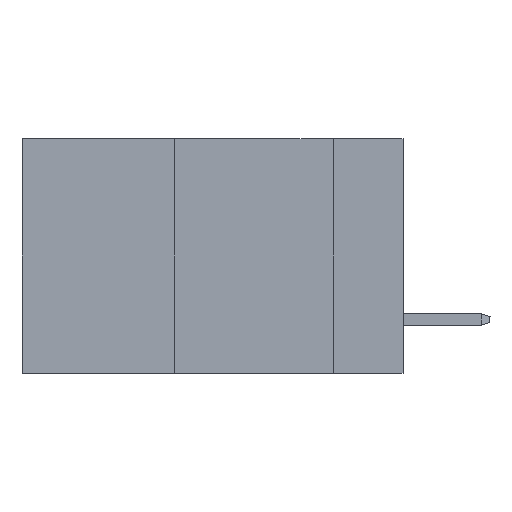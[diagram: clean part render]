
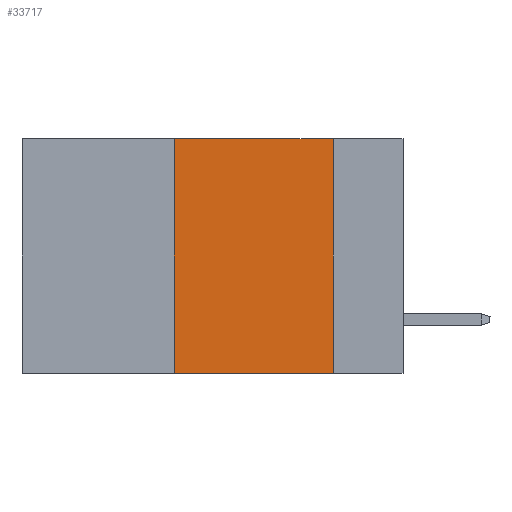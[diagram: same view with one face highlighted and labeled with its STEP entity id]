
A CAD part, left-side view. The second image highlights one B-rep face of the part: STEP entity #33717.
In plain terms, the highlighted planar face has unit normal (-1, 0, 0).
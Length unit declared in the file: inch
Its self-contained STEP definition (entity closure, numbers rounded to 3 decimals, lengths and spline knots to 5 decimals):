
#61 = VECTOR ( 'NONE', #30044, 39.37008 ) ;
#2435 = PLANE ( 'NONE',  #6922 ) ;
#2990 = FACE_OUTER_BOUND ( 'NONE', #19179, .T. ) ;
#3526 = VERTEX_POINT ( 'NONE', #31334 ) ;
#5348 = LINE ( 'NONE', #14117, #12496 ) ;
#5813 = CARTESIAN_POINT ( 'NONE',  ( 0., 0.36, -0.37 ) ) ;
#6833 = VECTOR ( 'NONE', #10161, 39.37008 ) ;
#6896 = CARTESIAN_POINT ( 'NONE',  ( 0., 0.11, 0. ) ) ;
#6922 = AXIS2_PLACEMENT_3D ( 'NONE', #34213, #17043, #23262 ) ;
#7102 = EDGE_CURVE ( 'NONE', #29738, #3526, #18357, .T. ) ;
#7328 = CARTESIAN_POINT ( 'NONE',  ( 0., 0.6, 0. ) ) ;
#10161 = DIRECTION ( 'NONE',  ( 0., -1., 0. ) ) ;
#10679 = ORIENTED_EDGE ( 'NONE', *, *, #21706, .F. ) ;
#11231 = DIRECTION ( 'NONE',  ( 0., 0., 1. ) ) ;
#12496 = VECTOR ( 'NONE', #11231, 39.37008 ) ;
#12799 = LINE ( 'NONE', #6896, #19404 ) ;
#14117 = CARTESIAN_POINT ( 'NONE',  ( 0., 0.36, 0. ) ) ;
#15057 = EDGE_CURVE ( 'NONE', #26358, #29738, #5348, .T. ) ;
#15480 = ORIENTED_EDGE ( 'NONE', *, *, #15057, .F. ) ;
#17043 = DIRECTION ( 'NONE',  ( 1., 0., 0. ) ) ;
#18123 = ORIENTED_EDGE ( 'NONE', *, *, #30701, .T. ) ;
#18357 = LINE ( 'NONE', #7328, #61 ) ;
#19179 = EDGE_LOOP ( 'NONE', ( #10679, #25588, #15480, #18123 ) ) ;
#19404 = VECTOR ( 'NONE', #32237, 39.37008 ) ;
#19827 = CARTESIAN_POINT ( 'NONE',  ( 0., 0.36, 0. ) ) ;
#20708 = CARTESIAN_POINT ( 'NONE',  ( 0., 0.11, -0.37 ) ) ;
#21706 = EDGE_CURVE ( 'NONE', #3526, #30285, #12799, .T. ) ;
#23262 = DIRECTION ( 'NONE',  ( 0., 0., -1. ) ) ;
#24020 = LINE ( 'NONE', #35705, #6833 ) ;
#25588 = ORIENTED_EDGE ( 'NONE', *, *, #7102, .F. ) ;
#26358 = VERTEX_POINT ( 'NONE', #5813 ) ;
#29738 = VERTEX_POINT ( 'NONE', #19827 ) ;
#30044 = DIRECTION ( 'NONE',  ( 0., -1., 0. ) ) ;
#30285 = VERTEX_POINT ( 'NONE', #20708 ) ;
#30701 = EDGE_CURVE ( 'NONE', #26358, #30285, #24020, .T. ) ;
#31334 = CARTESIAN_POINT ( 'NONE',  ( 0., 0.11, 0. ) ) ;
#32237 = DIRECTION ( 'NONE',  ( 0., 0., -1. ) ) ;
#33717 = ADVANCED_FACE ( 'NONE', ( #2990 ), #2435, .F. ) ;
#34213 = CARTESIAN_POINT ( 'NONE',  ( 0., 0.6, 0. ) ) ;
#35705 = CARTESIAN_POINT ( 'NONE',  ( 0., 0.6, -0.37 ) ) ;
